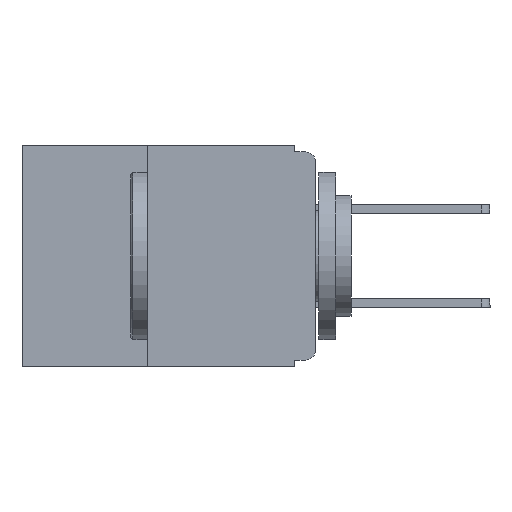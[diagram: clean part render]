
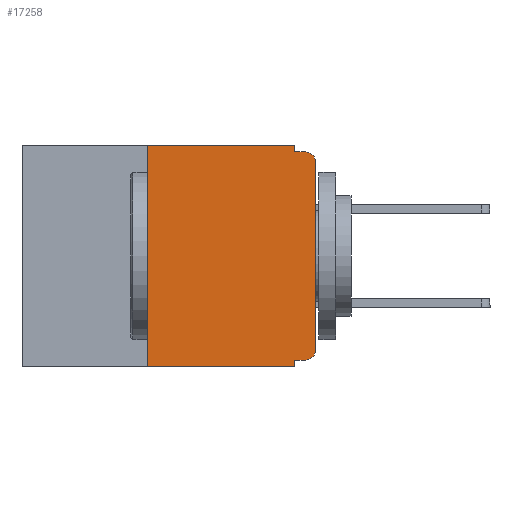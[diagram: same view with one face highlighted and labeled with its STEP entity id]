
A CAD part, left-side view. The second image highlights one B-rep face of the part: STEP entity #17258.
In plain terms, the highlighted planar face has unit normal (-1, 0, 0).
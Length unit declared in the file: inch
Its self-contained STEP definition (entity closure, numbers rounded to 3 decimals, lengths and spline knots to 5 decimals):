
#46 = DIRECTION ( 'NONE',  ( 1., 0., 0. ) ) ;
#146 = CARTESIAN_POINT ( 'NONE',  ( 0., 0.031, -0.32 ) ) ;
#216 = EDGE_CURVE ( 'NONE', #20004, #3927, #13975, .T. ) ;
#631 = VECTOR ( 'NONE', #10631, 39.37008 ) ;
#889 = CARTESIAN_POINT ( 'NONE',  ( 0., 0.031, -0.01 ) ) ;
#1138 = VERTEX_POINT ( 'NONE', #10734 ) ;
#1253 = ORIENTED_EDGE ( 'NONE', *, *, #9988, .T. ) ;
#1283 = LINE ( 'NONE', #20197, #631 ) ;
#1593 = CARTESIAN_POINT ( 'NONE',  ( 0., 0.031, 0. ) ) ;
#1676 = DIRECTION ( 'NONE',  ( 0., -1., 0. ) ) ;
#2486 = LINE ( 'NONE', #23325, #11715 ) ;
#2688 = CARTESIAN_POINT ( 'NONE',  ( 0., 0.437, 0. ) ) ;
#2930 = CARTESIAN_POINT ( 'NONE',  ( 0., 0.015, -0.32 ) ) ;
#3630 = VERTEX_POINT ( 'NONE', #1593 ) ;
#3927 = VERTEX_POINT ( 'NONE', #11595 ) ;
#4125 = LINE ( 'NONE', #14566, #13901 ) ;
#4128 = DIRECTION ( 'NONE',  ( 0., -1., 0. ) ) ;
#4644 = VECTOR ( 'NONE', #1676, 39.37008 ) ;
#4669 = DIRECTION ( 'NONE',  ( 0., -1., 0. ) ) ;
#5865 = VERTEX_POINT ( 'NONE', #21021 ) ;
#6015 = EDGE_CURVE ( 'NONE', #19400, #20004, #20474, .T. ) ;
#6074 = VECTOR ( 'NONE', #14468, 39.37008 ) ;
#6369 = DIRECTION ( 'NONE',  ( 0., 0., 1. ) ) ;
#7129 = ORIENTED_EDGE ( 'NONE', *, *, #18998, .F. ) ;
#7644 = CARTESIAN_POINT ( 'NONE',  ( 0., 0., -0.01 ) ) ;
#7767 = ORIENTED_EDGE ( 'NONE', *, *, #17517, .F. ) ;
#7939 = CARTESIAN_POINT ( 'NONE',  ( 0., 0.437, 0. ) ) ;
#8836 = LINE ( 'NONE', #2688, #13367 ) ;
#9309 = CARTESIAN_POINT ( 'NONE',  ( 0., 0.015, -0.025 ) ) ;
#9685 = CARTESIAN_POINT ( 'NONE',  ( 0., 0.031, -0.33 ) ) ;
#9988 = EDGE_CURVE ( 'NONE', #3927, #19551, #23200, .T. ) ;
#10295 = FACE_OUTER_BOUND ( 'NONE', #18340, .T. ) ;
#10543 = AXIS2_PLACEMENT_3D ( 'NONE', #15580, #15500, #15376 ) ;
#10631 = DIRECTION ( 'NONE',  ( 0., 1., 0. ) ) ;
#10734 = CARTESIAN_POINT ( 'NONE',  ( 0., 0.25, -0.33 ) ) ;
#10809 = ORIENTED_EDGE ( 'NONE', *, *, #12373, .F. ) ;
#11250 = DIRECTION ( 'NONE',  ( 0., 0., -1. ) ) ;
#11309 = VERTEX_POINT ( 'NONE', #9685 ) ;
#11361 = CARTESIAN_POINT ( 'NONE',  ( 0., 0.015, -0.01 ) ) ;
#11595 = CARTESIAN_POINT ( 'NONE',  ( 0., 0., -0.025 ) ) ;
#11715 = VECTOR ( 'NONE', #4128, 39.37008 ) ;
#11733 = ORIENTED_EDGE ( 'NONE', *, *, #6015, .T. ) ;
#12373 = EDGE_CURVE ( 'NONE', #16318, #11309, #15925, .T. ) ;
#12571 = EDGE_CURVE ( 'NONE', #19400, #16318, #1283, .T. ) ;
#13367 = VECTOR ( 'NONE', #4669, 39.37008 ) ;
#13650 = EDGE_CURVE ( 'NONE', #1138, #11309, #2486, .T. ) ;
#13769 = DIRECTION ( 'NONE',  ( 0., 0., -1. ) ) ;
#13901 = VECTOR ( 'NONE', #16522, 39.37008 ) ;
#13919 = CARTESIAN_POINT ( 'NONE',  ( 0., 0.031, -0.33 ) ) ;
#13975 = LINE ( 'NONE', #18659, #6074 ) ;
#14097 = ORIENTED_EDGE ( 'NONE', *, *, #14933, .F. ) ;
#14468 = DIRECTION ( 'NONE',  ( 0., 0., 1. ) ) ;
#14566 = CARTESIAN_POINT ( 'NONE',  ( 0., 0.031, 0. ) ) ;
#14580 = AXIS2_PLACEMENT_3D ( 'NONE', #7939, #46, #13769 ) ;
#14933 = EDGE_CURVE ( 'NONE', #1138, #5865, #18547, .T. ) ;
#15376 = DIRECTION ( 'NONE',  ( 0., 0., -1. ) ) ;
#15500 = DIRECTION ( 'NONE',  ( -1., 0., 0. ) ) ;
#15580 = CARTESIAN_POINT ( 'NONE',  ( 0., 0.015, -0.305 ) ) ;
#15925 = LINE ( 'NONE', #13919, #21040 ) ;
#16027 = CARTESIAN_POINT ( 'NONE',  ( 0., 0.25, -0.33 ) ) ;
#16318 = VERTEX_POINT ( 'NONE', #146 ) ;
#16522 = DIRECTION ( 'NONE',  ( 0., 0., -1. ) ) ;
#17130 = ORIENTED_EDGE ( 'NONE', *, *, #12571, .F. ) ;
#17258 = ADVANCED_FACE ( 'NONE', ( #10295 ), #23229, .F. ) ;
#17517 = EDGE_CURVE ( 'NONE', #3630, #20625, #4125, .T. ) ;
#17939 = VECTOR ( 'NONE', #6369, 39.37008 ) ;
#18340 = EDGE_LOOP ( 'NONE', ( #21296, #1253, #7129, #7767, #23026, #14097, #19218, #10809, #17130, #11733 ) ) ;
#18455 = CARTESIAN_POINT ( 'NONE',  ( 0., 0., -0.305 ) ) ;
#18547 = LINE ( 'NONE', #16027, #17939 ) ;
#18659 = CARTESIAN_POINT ( 'NONE',  ( 0., 0., 0. ) ) ;
#18998 = EDGE_CURVE ( 'NONE', #20625, #19551, #19513, .T. ) ;
#19218 = ORIENTED_EDGE ( 'NONE', *, *, #13650, .T. ) ;
#19400 = VERTEX_POINT ( 'NONE', #2930 ) ;
#19513 = LINE ( 'NONE', #7644, #4644 ) ;
#19551 = VERTEX_POINT ( 'NONE', #11361 ) ;
#20004 = VERTEX_POINT ( 'NONE', #18455 ) ;
#20197 = CARTESIAN_POINT ( 'NONE',  ( 0., 0., -0.32 ) ) ;
#20474 = CIRCLE ( 'NONE', #10543, 0.015 ) ;
#20625 = VERTEX_POINT ( 'NONE', #889 ) ;
#21021 = CARTESIAN_POINT ( 'NONE',  ( 0., 0.25, 0. ) ) ;
#21040 = VECTOR ( 'NONE', #23305, 39.37008 ) ;
#21296 = ORIENTED_EDGE ( 'NONE', *, *, #216, .T. ) ;
#21437 = EDGE_CURVE ( 'NONE', #5865, #3630, #8836, .T. ) ;
#22675 = DIRECTION ( 'NONE',  ( -1., 0., 0. ) ) ;
#23026 = ORIENTED_EDGE ( 'NONE', *, *, #21437, .F. ) ;
#23200 = CIRCLE ( 'NONE', #23517, 0.015 ) ;
#23229 = PLANE ( 'NONE',  #14580 ) ;
#23305 = DIRECTION ( 'NONE',  ( 0., 0., -1. ) ) ;
#23325 = CARTESIAN_POINT ( 'NONE',  ( 0., 0.437, -0.33 ) ) ;
#23517 = AXIS2_PLACEMENT_3D ( 'NONE', #9309, #22675, #11250 ) ;
